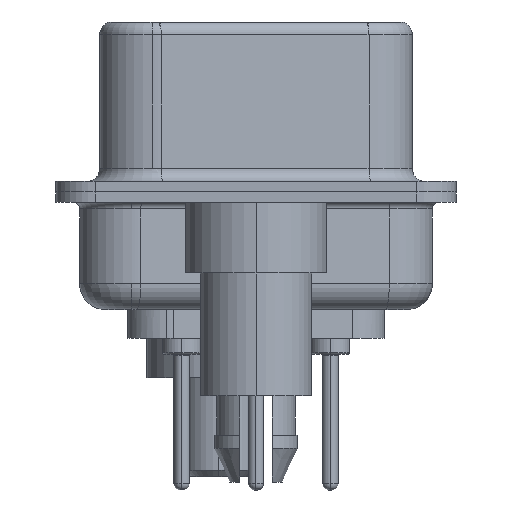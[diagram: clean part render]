
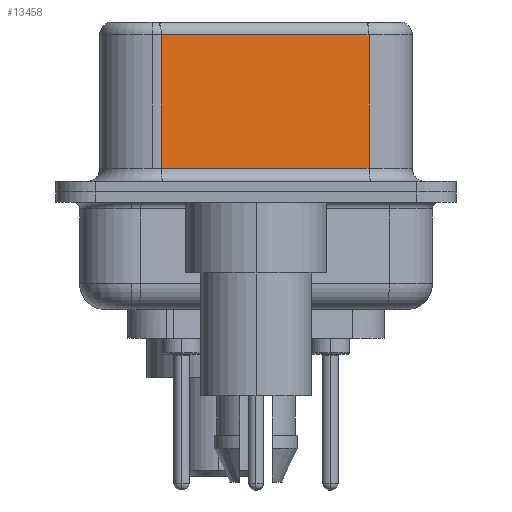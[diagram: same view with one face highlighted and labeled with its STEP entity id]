
A CAD part, left-side view. The second image highlights one B-rep face of the part: STEP entity #13458.
In plain terms, the highlighted planar face has unit normal (-0.985, -0.174, 0).
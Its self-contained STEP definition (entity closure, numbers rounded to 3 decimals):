
#9 = VECTOR ( 'NONE', #11666, 1000. ) ;
#136 = EDGE_CURVE ( 'NONE', #1583, #16242, #15584, .T. ) ;
#484 = AXIS2_PLACEMENT_3D ( 'NONE', #12356, #14709, #973 ) ;
#867 = PLANE ( 'NONE',  #484 ) ;
#973 = DIRECTION ( 'NONE',  ( -0.174, 0.985, 0. ) ) ;
#1285 = LINE ( 'NONE', #15196, #2431 ) ;
#1535 = EDGE_CURVE ( 'NONE', #1583, #2784, #21754, .T. ) ;
#1583 = VERTEX_POINT ( 'NONE', #16503 ) ;
#2189 = ORIENTED_EDGE ( 'NONE', *, *, #19512, .T. ) ;
#2431 = VECTOR ( 'NONE', #20488, 1000. ) ;
#2718 = DIRECTION ( 'NONE',  ( 0., 0., -1. ) ) ;
#2784 = VERTEX_POINT ( 'NONE', #25779 ) ;
#6226 = DIRECTION ( 'NONE',  ( -0.174, 0.985, 0. ) ) ;
#7086 = VECTOR ( 'NONE', #2718, 1000. ) ;
#7135 = CARTESIAN_POINT ( 'NONE',  ( 5.132, -4.322, 6.52 ) ) ;
#9390 = VECTOR ( 'NONE', #6226, 1000. ) ;
#11666 = DIRECTION ( 'NONE',  ( 0.174, -0.985, 0. ) ) ;
#12015 = ORIENTED_EDGE ( 'NONE', *, *, #1535, .F. ) ;
#12356 = CARTESIAN_POINT ( 'NONE',  ( 5.132, -4.322, 6.52 ) ) ;
#13458 = ADVANCED_FACE ( 'NONE', ( #26455 ), #867, .F. ) ;
#14709 = DIRECTION ( 'NONE',  ( 0.985, 0.174, 0. ) ) ;
#15196 = CARTESIAN_POINT ( 'NONE',  ( 3.73, 3.628, 6.52 ) ) ;
#15584 = LINE ( 'NONE', #29286, #9390 ) ;
#15917 = EDGE_CURVE ( 'NONE', #16242, #29023, #1285, .T. ) ;
#16043 = CARTESIAN_POINT ( 'NONE',  ( 3.73, 3.628, 0.9 ) ) ;
#16163 = ORIENTED_EDGE ( 'NONE', *, *, #15917, .T. ) ;
#16242 = VERTEX_POINT ( 'NONE', #18272 ) ;
#16503 = CARTESIAN_POINT ( 'NONE',  ( 5.132, -4.322, 6.02 ) ) ;
#18272 = CARTESIAN_POINT ( 'NONE',  ( 3.73, 3.628, 6.02 ) ) ;
#18352 = LINE ( 'NONE', #23487, #9 ) ;
#19512 = EDGE_CURVE ( 'NONE', #29023, #2784, #18352, .T. ) ;
#20488 = DIRECTION ( 'NONE',  ( 0., 0., -1. ) ) ;
#20556 = ORIENTED_EDGE ( 'NONE', *, *, #136, .T. ) ;
#21754 = LINE ( 'NONE', #7135, #7086 ) ;
#23487 = CARTESIAN_POINT ( 'NONE',  ( 5.132, -4.322, 0.9 ) ) ;
#24077 = EDGE_LOOP ( 'NONE', ( #12015, #20556, #16163, #2189 ) ) ;
#25779 = CARTESIAN_POINT ( 'NONE',  ( 5.132, -4.322, 0.9 ) ) ;
#26455 = FACE_OUTER_BOUND ( 'NONE', #24077, .T. ) ;
#29023 = VERTEX_POINT ( 'NONE', #16043 ) ;
#29286 = CARTESIAN_POINT ( 'NONE',  ( 5.132, -4.322, 6.02 ) ) ;
